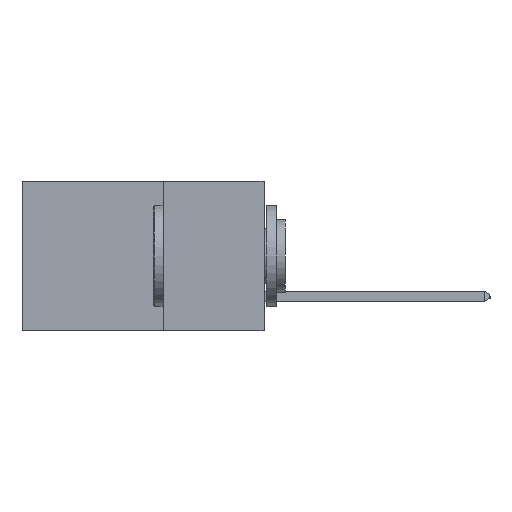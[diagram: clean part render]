
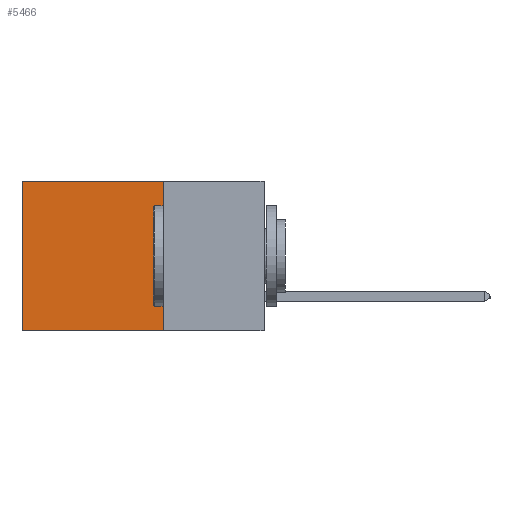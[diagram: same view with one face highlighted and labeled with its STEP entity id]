
A CAD part, left-side view. The second image highlights one B-rep face of the part: STEP entity #5466.
In plain terms, the highlighted planar face has unit normal (-1, 0, 0).
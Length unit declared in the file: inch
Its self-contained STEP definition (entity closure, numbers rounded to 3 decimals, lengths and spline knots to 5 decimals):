
#849 = EDGE_CURVE ( 'NONE', #16274, #13071, #2048, .T. ) ;
#1179 = CARTESIAN_POINT ( 'NONE',  ( 0.298, 0.6, -0.37 ) ) ;
#1907 = EDGE_LOOP ( 'NONE', ( #18980, #20648, #15576, #3389 ) ) ;
#2048 = LINE ( 'NONE', #9982, #19635 ) ;
#3083 = EDGE_CURVE ( 'NONE', #16274, #5342, #18522, .T. ) ;
#3286 = LINE ( 'NONE', #5561, #16348 ) ;
#3389 = ORIENTED_EDGE ( 'NONE', *, *, #3083, .T. ) ;
#4655 = CARTESIAN_POINT ( 'NONE',  ( 0.298, 0.25, 0. ) ) ;
#5342 = VERTEX_POINT ( 'NONE', #21326 ) ;
#5466 = ADVANCED_FACE ( 'NONE', ( #18134 ), #14875, .F. ) ;
#5561 = CARTESIAN_POINT ( 'NONE',  ( 0.298, 0.25, -0.37 ) ) ;
#5786 = CARTESIAN_POINT ( 'NONE',  ( 0.298, 0.25, -0.37 ) ) ;
#6349 = DIRECTION ( 'NONE',  ( 0., 0., -1. ) ) ;
#7612 = DIRECTION ( 'NONE',  ( 0., 0., -1. ) ) ;
#9025 = DIRECTION ( 'NONE',  ( 0., 1., 0. ) ) ;
#9320 = CARTESIAN_POINT ( 'NONE',  ( 0.298, 0.6, 0. ) ) ;
#9469 = CARTESIAN_POINT ( 'NONE',  ( 0.298, 0.25, 0. ) ) ;
#9979 = VERTEX_POINT ( 'NONE', #1179 ) ;
#9982 = CARTESIAN_POINT ( 'NONE',  ( 0.298, 0.25, 0. ) ) ;
#10262 = LINE ( 'NONE', #9320, #15294 ) ;
#11747 = EDGE_CURVE ( 'NONE', #13071, #9979, #3286, .T. ) ;
#11826 = EDGE_CURVE ( 'NONE', #5342, #9979, #10262, .T. ) ;
#13071 = VERTEX_POINT ( 'NONE', #5786 ) ;
#14004 = AXIS2_PLACEMENT_3D ( 'NONE', #4655, #16568, #6349 ) ;
#14043 = VECTOR ( 'NONE', #15258, 39.37008 ) ;
#14875 = PLANE ( 'NONE',  #14004 ) ;
#15258 = DIRECTION ( 'NONE',  ( 0., 1., 0. ) ) ;
#15294 = VECTOR ( 'NONE', #21183, 39.37008 ) ;
#15357 = CARTESIAN_POINT ( 'NONE',  ( 0.298, 0.25, 0. ) ) ;
#15576 = ORIENTED_EDGE ( 'NONE', *, *, #849, .F. ) ;
#16274 = VERTEX_POINT ( 'NONE', #9469 ) ;
#16348 = VECTOR ( 'NONE', #9025, 39.37008 ) ;
#16568 = DIRECTION ( 'NONE',  ( 1., 0., 0. ) ) ;
#18134 = FACE_OUTER_BOUND ( 'NONE', #1907, .T. ) ;
#18522 = LINE ( 'NONE', #15357, #14043 ) ;
#18980 = ORIENTED_EDGE ( 'NONE', *, *, #11826, .T. ) ;
#19635 = VECTOR ( 'NONE', #7612, 39.37008 ) ;
#20648 = ORIENTED_EDGE ( 'NONE', *, *, #11747, .F. ) ;
#21183 = DIRECTION ( 'NONE',  ( 0., 0., -1. ) ) ;
#21326 = CARTESIAN_POINT ( 'NONE',  ( 0.298, 0.6, 0. ) ) ;
